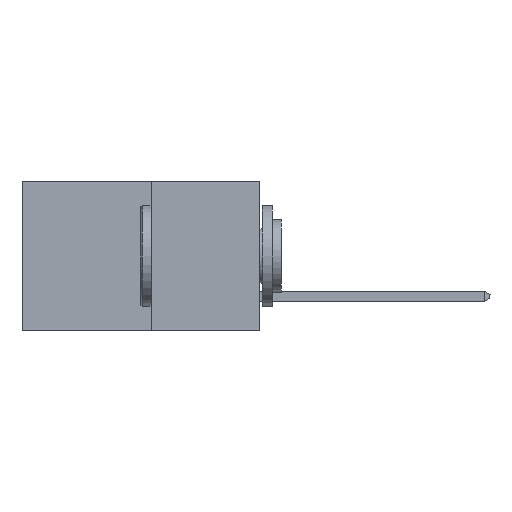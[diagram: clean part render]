
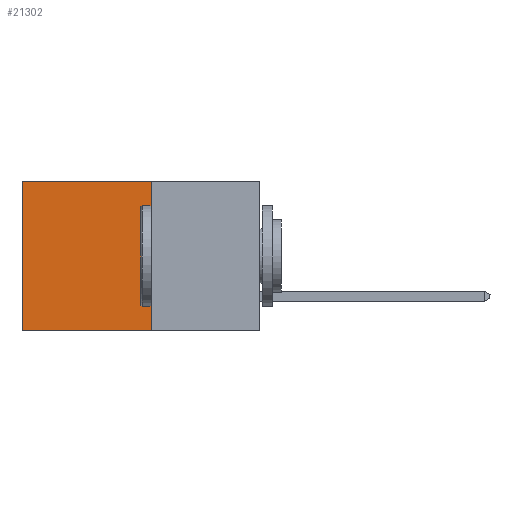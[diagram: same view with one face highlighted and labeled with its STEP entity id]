
A CAD part, left-side view. The second image highlights one B-rep face of the part: STEP entity #21302.
In plain terms, the highlighted planar face has unit normal (-1, 0, 0).
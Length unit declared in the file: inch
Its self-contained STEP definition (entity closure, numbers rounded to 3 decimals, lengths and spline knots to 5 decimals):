
#516 = DIRECTION ( 'NONE',  ( 0., 0., -1. ) ) ;
#961 = DIRECTION ( 'NONE',  ( 0., 1., 0. ) ) ;
#3584 = LINE ( 'NONE', #13159, #13386 ) ;
#3771 = VECTOR ( 'NONE', #961, 39.37008 ) ;
#4025 = CARTESIAN_POINT ( 'NONE',  ( 0.277, 0.59, -0.37 ) ) ;
#4729 = PLANE ( 'NONE',  #16133 ) ;
#5046 = ORIENTED_EDGE ( 'NONE', *, *, #5199, .T. ) ;
#5199 = EDGE_CURVE ( 'NONE', #13556, #16767, #24991, .T. ) ;
#5392 = ORIENTED_EDGE ( 'NONE', *, *, #5465, .F. ) ;
#5465 = EDGE_CURVE ( 'NONE', #18649, #14179, #10074, .T. ) ;
#5724 = ORIENTED_EDGE ( 'NONE', *, *, #9443, .T. ) ;
#6921 = DIRECTION ( 'NONE',  ( 0., 0., -1. ) ) ;
#9443 = EDGE_CURVE ( 'NONE', #16767, #14179, #3584, .T. ) ;
#10074 = LINE ( 'NONE', #10253, #25661 ) ;
#10253 = CARTESIAN_POINT ( 'NONE',  ( 0.277, 0.27, -0.37 ) ) ;
#10695 = CARTESIAN_POINT ( 'NONE',  ( 0.277, 0.27, -0.37 ) ) ;
#11610 = LINE ( 'NONE', #17029, #16448 ) ;
#13090 = DIRECTION ( 'NONE',  ( 1., 0., 0. ) ) ;
#13159 = CARTESIAN_POINT ( 'NONE',  ( 0.277, 0.59, -0.37 ) ) ;
#13386 = VECTOR ( 'NONE', #6921, 39.37008 ) ;
#13556 = VERTEX_POINT ( 'NONE', #16405 ) ;
#14179 = VERTEX_POINT ( 'NONE', #4025 ) ;
#16133 = AXIS2_PLACEMENT_3D ( 'NONE', #25240, #13090, #516 ) ;
#16405 = CARTESIAN_POINT ( 'NONE',  ( 0.277, 0.27, 0. ) ) ;
#16448 = VECTOR ( 'NONE', #23002, 39.37008 ) ;
#16767 = VERTEX_POINT ( 'NONE', #22848 ) ;
#17029 = CARTESIAN_POINT ( 'NONE',  ( 0.277, 0.27, -0.37 ) ) ;
#17606 = CARTESIAN_POINT ( 'NONE',  ( 0.277, 0.27, 0. ) ) ;
#18649 = VERTEX_POINT ( 'NONE', #10695 ) ;
#19119 = ORIENTED_EDGE ( 'NONE', *, *, #22625, .F. ) ;
#19273 = EDGE_LOOP ( 'NONE', ( #5724, #5392, #19119, #5046 ) ) ;
#20470 = DIRECTION ( 'NONE',  ( 0., 1., 0. ) ) ;
#21302 = ADVANCED_FACE ( 'NONE', ( #23203 ), #4729, .F. ) ;
#22625 = EDGE_CURVE ( 'NONE', #13556, #18649, #11610, .T. ) ;
#22848 = CARTESIAN_POINT ( 'NONE',  ( 0.277, 0.59, 0. ) ) ;
#23002 = DIRECTION ( 'NONE',  ( 0., 0., -1. ) ) ;
#23203 = FACE_OUTER_BOUND ( 'NONE', #19273, .T. ) ;
#24991 = LINE ( 'NONE', #17606, #3771 ) ;
#25240 = CARTESIAN_POINT ( 'NONE',  ( 0.277, 0.27, -0.37 ) ) ;
#25661 = VECTOR ( 'NONE', #20470, 39.37008 ) ;
